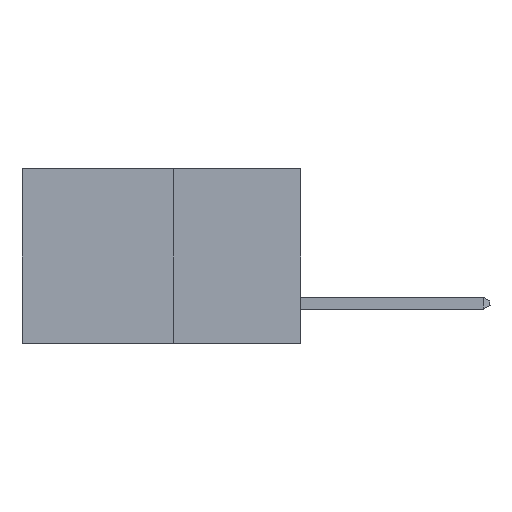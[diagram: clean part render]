
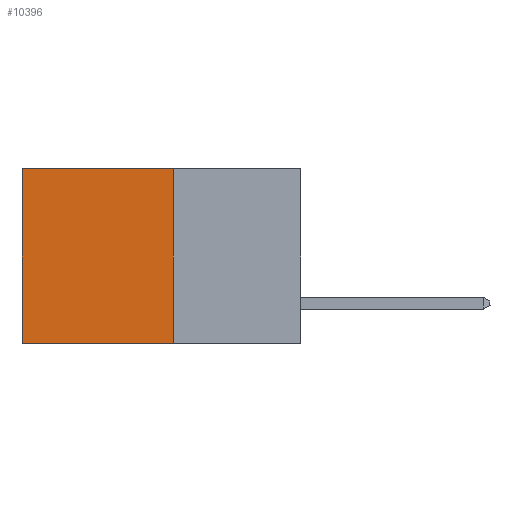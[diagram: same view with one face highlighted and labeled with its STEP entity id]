
A CAD part, left-side view. The second image highlights one B-rep face of the part: STEP entity #10396.
In plain terms, the highlighted planar face has unit normal (-1, 0, 0).
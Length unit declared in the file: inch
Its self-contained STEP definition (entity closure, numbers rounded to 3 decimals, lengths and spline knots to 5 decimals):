
#729 = VERTEX_POINT ( 'NONE', #3505 ) ;
#864 = VERTEX_POINT ( 'NONE', #10103 ) ;
#2470 = LINE ( 'NONE', #12894, #12086 ) ;
#3106 = EDGE_LOOP ( 'NONE', ( #14968, #4080, #9086, #9962 ) ) ;
#3468 = DIRECTION ( 'NONE',  ( 0., 1., 0. ) ) ;
#3505 = CARTESIAN_POINT ( 'NONE',  ( 0.277, 0.27, 0. ) ) ;
#3739 = FACE_OUTER_BOUND ( 'NONE', #3106, .T. ) ;
#4080 = ORIENTED_EDGE ( 'NONE', *, *, #14026, .F. ) ;
#4494 = LINE ( 'NONE', #11855, #13473 ) ;
#4634 = CARTESIAN_POINT ( 'NONE',  ( 0.277, 0.27, -0.37 ) ) ;
#5851 = DIRECTION ( 'NONE',  ( 0., 0., -1. ) ) ;
#5863 = LINE ( 'NONE', #11860, #11802 ) ;
#7042 = EDGE_CURVE ( 'NONE', #729, #864, #2470, .T. ) ;
#7233 = LINE ( 'NONE', #9494, #10104 ) ;
#7479 = VERTEX_POINT ( 'NONE', #12504 ) ;
#8008 = CARTESIAN_POINT ( 'NONE',  ( 0.277, 0.59, -0.37 ) ) ;
#8075 = AXIS2_PLACEMENT_3D ( 'NONE', #4634, #12876, #5851 ) ;
#9086 = ORIENTED_EDGE ( 'NONE', *, *, #7042, .F. ) ;
#9494 = CARTESIAN_POINT ( 'NONE',  ( 0.277, 0.59, -0.37 ) ) ;
#9962 = ORIENTED_EDGE ( 'NONE', *, *, #10457, .T. ) ;
#10103 = CARTESIAN_POINT ( 'NONE',  ( 0.277, 0.27, -0.37 ) ) ;
#10104 = VECTOR ( 'NONE', #10632, 39.37008 ) ;
#10396 = ADVANCED_FACE ( 'NONE', ( #3739 ), #11765, .F. ) ;
#10457 = EDGE_CURVE ( 'NONE', #729, #7479, #5863, .T. ) ;
#10632 = DIRECTION ( 'NONE',  ( 0., 0., -1. ) ) ;
#11765 = PLANE ( 'NONE',  #8075 ) ;
#11802 = VECTOR ( 'NONE', #12973, 39.37008 ) ;
#11855 = CARTESIAN_POINT ( 'NONE',  ( 0.277, 0.27, -0.37 ) ) ;
#11860 = CARTESIAN_POINT ( 'NONE',  ( 0.277, 0.27, 0. ) ) ;
#12086 = VECTOR ( 'NONE', #13992, 39.37008 ) ;
#12504 = CARTESIAN_POINT ( 'NONE',  ( 0.277, 0.59, 0. ) ) ;
#12876 = DIRECTION ( 'NONE',  ( 1., 0., 0. ) ) ;
#12894 = CARTESIAN_POINT ( 'NONE',  ( 0.277, 0.27, -0.37 ) ) ;
#12973 = DIRECTION ( 'NONE',  ( 0., 1., 0. ) ) ;
#13473 = VECTOR ( 'NONE', #3468, 39.37008 ) ;
#13950 = VERTEX_POINT ( 'NONE', #8008 ) ;
#13992 = DIRECTION ( 'NONE',  ( 0., 0., -1. ) ) ;
#14026 = EDGE_CURVE ( 'NONE', #864, #13950, #4494, .T. ) ;
#14029 = EDGE_CURVE ( 'NONE', #7479, #13950, #7233, .T. ) ;
#14968 = ORIENTED_EDGE ( 'NONE', *, *, #14029, .T. ) ;
